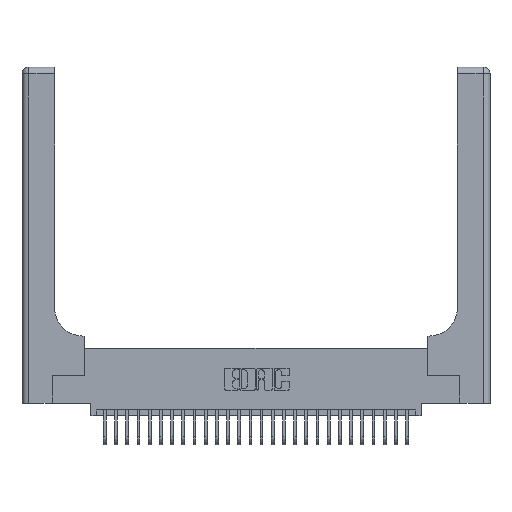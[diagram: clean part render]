
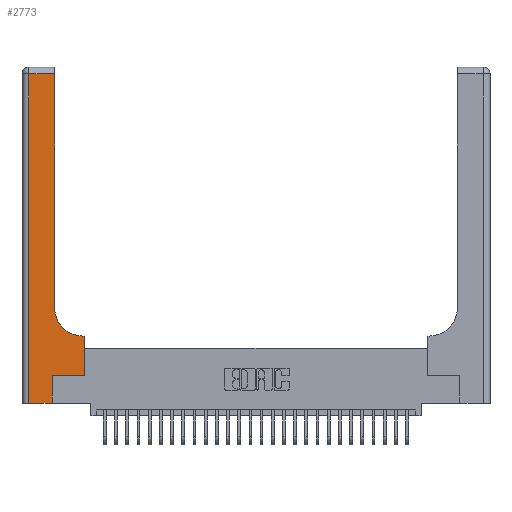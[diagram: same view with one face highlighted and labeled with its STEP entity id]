
A CAD part, top view. The second image highlights one B-rep face of the part: STEP entity #2773.
In plain terms, the highlighted planar face has unit normal (0, 0, 1).
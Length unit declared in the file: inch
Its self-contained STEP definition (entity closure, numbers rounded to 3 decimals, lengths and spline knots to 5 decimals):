
#700 = CARTESIAN_POINT ( 'NONE',  ( 0.269, 0.25, 0.37 ) ) ;
#1538 = EDGE_CURVE ( 'NONE', #26719, #9871, #4741, .T. ) ;
#2374 = EDGE_LOOP ( 'NONE', ( #18204, #10798, #4454, #7894, #16738, #6101, #18987, #10317, #5221 ) ) ;
#2572 = DIRECTION ( 'NONE',  ( 0., 0., -1. ) ) ;
#2696 = EDGE_CURVE ( 'NONE', #8718, #8442, #25933, .T. ) ;
#2773 = ADVANCED_FACE ( 'NONE', ( #23211 ), #9099, .F. ) ;
#4371 = CIRCLE ( 'NONE', #11482, 0.25 ) ;
#4454 = ORIENTED_EDGE ( 'NONE', *, *, #1538, .T. ) ;
#4576 = VERTEX_POINT ( 'NONE', #27891 ) ;
#4741 = LINE ( 'NONE', #26542, #27996 ) ;
#4933 = DIRECTION ( 'NONE',  ( 0., 1., 0. ) ) ;
#5221 = ORIENTED_EDGE ( 'NONE', *, *, #7097, .T. ) ;
#5535 = DIRECTION ( 'NONE',  ( 1., 0., 0. ) ) ;
#5853 = CARTESIAN_POINT ( 'NONE',  ( 0.5585, 0.25, 0.37 ) ) ;
#6101 = ORIENTED_EDGE ( 'NONE', *, *, #9790, .T. ) ;
#6958 = CARTESIAN_POINT ( 'NONE',  ( 0., 2.94, 0.37 ) ) ;
#7097 = EDGE_CURVE ( 'NONE', #8442, #20445, #4371, .T. ) ;
#7161 = CARTESIAN_POINT ( 'NONE',  ( 0.269, 0., 0.37 ) ) ;
#7345 = LINE ( 'NONE', #13241, #24116 ) ;
#7565 = LINE ( 'NONE', #27430, #25015 ) ;
#7894 = ORIENTED_EDGE ( 'NONE', *, *, #18960, .T. ) ;
#8442 = VERTEX_POINT ( 'NONE', #9851 ) ;
#8502 = VECTOR ( 'NONE', #11015, 39.37008 ) ;
#8569 = CARTESIAN_POINT ( 'NONE',  ( 0.5415, 0.85, 0.37 ) ) ;
#8718 = VERTEX_POINT ( 'NONE', #17294 ) ;
#8944 = EDGE_CURVE ( 'NONE', #4576, #23540, #15201, .T. ) ;
#9099 = PLANE ( 'NONE',  #9582 ) ;
#9453 = EDGE_CURVE ( 'NONE', #20445, #26970, #7345, .T. ) ;
#9582 = AXIS2_PLACEMENT_3D ( 'NONE', #15658, #2572, #17883 ) ;
#9790 = EDGE_CURVE ( 'NONE', #23540, #13322, #27495, .T. ) ;
#9851 = CARTESIAN_POINT ( 'NONE',  ( 0.5415, 0.6, 0.37 ) ) ;
#9871 = VERTEX_POINT ( 'NONE', #25361 ) ;
#10317 = ORIENTED_EDGE ( 'NONE', *, *, #2696, .T. ) ;
#10711 = CARTESIAN_POINT ( 'NONE',  ( 0.5585, 0.25, 0.37 ) ) ;
#10765 = DIRECTION ( 'NONE',  ( 1., 0., 0. ) ) ;
#10798 = ORIENTED_EDGE ( 'NONE', *, *, #15920, .T. ) ;
#11015 = DIRECTION ( 'NONE',  ( -1., 0., 0. ) ) ;
#11257 = DIRECTION ( 'NONE',  ( 0., -1., 0. ) ) ;
#11482 = AXIS2_PLACEMENT_3D ( 'NONE', #8569, #23885, #10765 ) ;
#13241 = CARTESIAN_POINT ( 'NONE',  ( 0.2915, 3., 0.37 ) ) ;
#13322 = VERTEX_POINT ( 'NONE', #10711 ) ;
#15201 = LINE ( 'NONE', #7161, #19693 ) ;
#15268 = CARTESIAN_POINT ( 'NONE',  ( 0.2915, 0.6, 0.37 ) ) ;
#15410 = DIRECTION ( 'NONE',  ( 0., 1., 0. ) ) ;
#15658 = CARTESIAN_POINT ( 'NONE',  ( 0., 3., 0.37 ) ) ;
#15726 = DIRECTION ( 'NONE',  ( -1., 0., 0. ) ) ;
#15920 = EDGE_CURVE ( 'NONE', #26970, #26719, #28182, .T. ) ;
#16738 = ORIENTED_EDGE ( 'NONE', *, *, #8944, .T. ) ;
#17294 = CARTESIAN_POINT ( 'NONE',  ( 0.5585, 0.6, 0.37 ) ) ;
#17571 = CARTESIAN_POINT ( 'NONE',  ( 0.2915, 2.94, 0.37 ) ) ;
#17883 = DIRECTION ( 'NONE',  ( -1., 0., 0. ) ) ;
#18204 = ORIENTED_EDGE ( 'NONE', *, *, #9453, .T. ) ;
#18401 = EDGE_CURVE ( 'NONE', #13322, #8718, #22654, .T. ) ;
#18960 = EDGE_CURVE ( 'NONE', #9871, #4576, #7565, .T. ) ;
#18987 = ORIENTED_EDGE ( 'NONE', *, *, #18401, .T. ) ;
#19693 = VECTOR ( 'NONE', #4933, 39.37008 ) ;
#20445 = VERTEX_POINT ( 'NONE', #25915 ) ;
#21022 = VECTOR ( 'NONE', #27369, 39.37008 ) ;
#21974 = VECTOR ( 'NONE', #23362, 39.37008 ) ;
#22405 = VECTOR ( 'NONE', #15726, 39.37008 ) ;
#22654 = LINE ( 'NONE', #5853, #21974 ) ;
#23211 = FACE_OUTER_BOUND ( 'NONE', #2374, .T. ) ;
#23343 = CARTESIAN_POINT ( 'NONE',  ( 0.06, 2.94, 0.37 ) ) ;
#23362 = DIRECTION ( 'NONE',  ( 0., 1., 0. ) ) ;
#23540 = VERTEX_POINT ( 'NONE', #700 ) ;
#23885 = DIRECTION ( 'NONE',  ( 0., 0., -1. ) ) ;
#24116 = VECTOR ( 'NONE', #15410, 39.37008 ) ;
#25015 = VECTOR ( 'NONE', #5535, 39.37008 ) ;
#25361 = CARTESIAN_POINT ( 'NONE',  ( 0.06, 0., 0.37 ) ) ;
#25915 = CARTESIAN_POINT ( 'NONE',  ( 0.2915, 0.85, 0.37 ) ) ;
#25933 = LINE ( 'NONE', #15268, #8502 ) ;
#26542 = CARTESIAN_POINT ( 'NONE',  ( 0.06, 3., 0.37 ) ) ;
#26719 = VERTEX_POINT ( 'NONE', #23343 ) ;
#26970 = VERTEX_POINT ( 'NONE', #17571 ) ;
#27369 = DIRECTION ( 'NONE',  ( 1., 0., 0. ) ) ;
#27430 = CARTESIAN_POINT ( 'NONE',  ( 0., 0., 0.37 ) ) ;
#27468 = CARTESIAN_POINT ( 'NONE',  ( 0.269, 0.25, 0.37 ) ) ;
#27495 = LINE ( 'NONE', #27468, #21022 ) ;
#27891 = CARTESIAN_POINT ( 'NONE',  ( 0.269, 0., 0.37 ) ) ;
#27996 = VECTOR ( 'NONE', #11257, 39.37008 ) ;
#28182 = LINE ( 'NONE', #6958, #22405 ) ;
